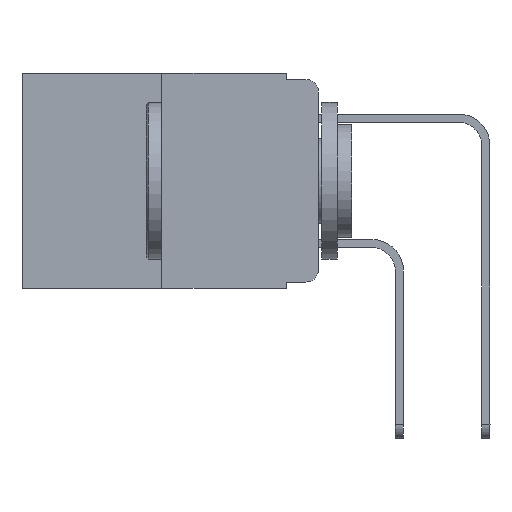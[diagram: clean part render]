
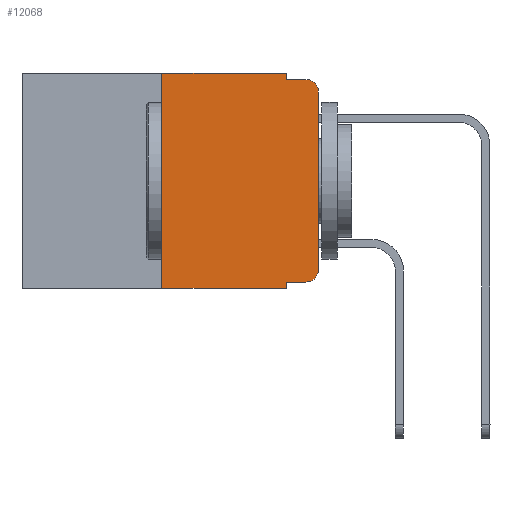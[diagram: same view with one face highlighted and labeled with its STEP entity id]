
A CAD part, left-side view. The second image highlights one B-rep face of the part: STEP entity #12068.
In plain terms, the highlighted planar face has unit normal (-1, 0, 0).
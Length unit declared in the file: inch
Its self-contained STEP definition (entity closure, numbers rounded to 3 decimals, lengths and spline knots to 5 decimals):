
#347 = CARTESIAN_POINT ( 'NONE',  ( 0., 0.051, -0.333 ) ) ;
#565 = LINE ( 'NONE', #16123, #12153 ) ;
#1091 = VERTEX_POINT ( 'NONE', #13543 ) ;
#1980 = DIRECTION ( 'NONE',  ( 0., 0., 1. ) ) ;
#3019 = DIRECTION ( 'NONE',  ( 0., 0., -1. ) ) ;
#3203 = PLANE ( 'NONE',  #16702 ) ;
#3685 = CARTESIAN_POINT ( 'NONE',  ( 0., 0.25, -0.343 ) ) ;
#3881 = DIRECTION ( 'NONE',  ( 0., 0., -1. ) ) ;
#3981 = ORIENTED_EDGE ( 'NONE', *, *, #6741, .F. ) ;
#4065 = VERTEX_POINT ( 'NONE', #16613 ) ;
#4074 = ORIENTED_EDGE ( 'NONE', *, *, #12992, .T. ) ;
#4576 = LINE ( 'NONE', #9655, #13757 ) ;
#4773 = ORIENTED_EDGE ( 'NONE', *, *, #21203, .T. ) ;
#4816 = AXIS2_PLACEMENT_3D ( 'NONE', #17775, #5701, #12593 ) ;
#5141 = CARTESIAN_POINT ( 'NONE',  ( 0., 0.02, -0.03 ) ) ;
#5701 = DIRECTION ( 'NONE',  ( -1., 0., 0. ) ) ;
#5902 = CARTESIAN_POINT ( 'NONE',  ( 0., 0.051, 0. ) ) ;
#6232 = VECTOR ( 'NONE', #3881, 39.37008 ) ;
#6681 = CARTESIAN_POINT ( 'NONE',  ( 0., 0., -0.313 ) ) ;
#6741 = EDGE_CURVE ( 'NONE', #17624, #17523, #10000, .T. ) ;
#6816 = ORIENTED_EDGE ( 'NONE', *, *, #11770, .F. ) ;
#6905 = DIRECTION ( 'NONE',  ( 0., 0., 1. ) ) ;
#7124 = CARTESIAN_POINT ( 'NONE',  ( 0., 0.25, 0. ) ) ;
#7152 = DIRECTION ( 'NONE',  ( 0., 0., -1. ) ) ;
#7201 = DIRECTION ( 'NONE',  ( 0., -1., 0. ) ) ;
#7350 = CIRCLE ( 'NONE', #18158, 0.02 ) ;
#7431 = DIRECTION ( 'NONE',  ( 0., -1., 0. ) ) ;
#8595 = DIRECTION ( 'NONE',  ( 0., 0., -1. ) ) ;
#8667 = ORIENTED_EDGE ( 'NONE', *, *, #10256, .F. ) ;
#8721 = ORIENTED_EDGE ( 'NONE', *, *, #20007, .T. ) ;
#8734 = EDGE_CURVE ( 'NONE', #21818, #17624, #14122, .T. ) ;
#8850 = DIRECTION ( 'NONE',  ( -1., 0., 0. ) ) ;
#9495 = ORIENTED_EDGE ( 'NONE', *, *, #8734, .F. ) ;
#9655 = CARTESIAN_POINT ( 'NONE',  ( 0., 0.051, -0.01 ) ) ;
#9665 = CARTESIAN_POINT ( 'NONE',  ( 0., 0., -0.03 ) ) ;
#9929 = VECTOR ( 'NONE', #1980, 39.37008 ) ;
#9994 = DIRECTION ( 'NONE',  ( 0., -1., 0. ) ) ;
#10000 = LINE ( 'NONE', #16873, #20249 ) ;
#10256 = EDGE_CURVE ( 'NONE', #12891, #20138, #4576, .T. ) ;
#10450 = VECTOR ( 'NONE', #6905, 39.37008 ) ;
#11178 = CARTESIAN_POINT ( 'NONE',  ( 0., 0.051, -0.333 ) ) ;
#11506 = VERTEX_POINT ( 'NONE', #9665 ) ;
#11571 = LINE ( 'NONE', #18458, #13852 ) ;
#11671 = DIRECTION ( 'NONE',  ( 0., -1., 0. ) ) ;
#11770 = EDGE_CURVE ( 'NONE', #12406, #1091, #12447, .T. ) ;
#12068 = ADVANCED_FACE ( 'NONE', ( #18648 ), #3203, .F. ) ;
#12153 = VECTOR ( 'NONE', #7431, 39.37008 ) ;
#12406 = VERTEX_POINT ( 'NONE', #11178 ) ;
#12447 = LINE ( 'NONE', #5902, #6232 ) ;
#12479 = VECTOR ( 'NONE', #7201, 39.37008 ) ;
#12593 = DIRECTION ( 'NONE',  ( 0., 0., -1. ) ) ;
#12862 = EDGE_CURVE ( 'NONE', #17523, #12891, #11571, .T. ) ;
#12891 = VERTEX_POINT ( 'NONE', #13718 ) ;
#12992 = EDGE_CURVE ( 'NONE', #11506, #20138, #7350, .T. ) ;
#13543 = CARTESIAN_POINT ( 'NONE',  ( 0., 0.051, -0.343 ) ) ;
#13711 = CARTESIAN_POINT ( 'NONE',  ( 0., 0., 0. ) ) ;
#13718 = CARTESIAN_POINT ( 'NONE',  ( 0., 0.051, -0.01 ) ) ;
#13757 = VECTOR ( 'NONE', #9994, 39.37008 ) ;
#13797 = CARTESIAN_POINT ( 'NONE',  ( 0., 0.473, 0. ) ) ;
#13852 = VECTOR ( 'NONE', #3019, 39.37008 ) ;
#13898 = DIRECTION ( 'NONE',  ( 1., 0., 0. ) ) ;
#14122 = LINE ( 'NONE', #7124, #10450 ) ;
#14223 = EDGE_LOOP ( 'NONE', ( #17016, #4074, #8667, #16635, #3981, #9495, #4773, #6816, #8721, #17682 ) ) ;
#15985 = EDGE_CURVE ( 'NONE', #4065, #19404, #20661, .T. ) ;
#16123 = CARTESIAN_POINT ( 'NONE',  ( 0., 0.473, -0.343 ) ) ;
#16548 = CARTESIAN_POINT ( 'NONE',  ( 0., 0.02, -0.01 ) ) ;
#16613 = CARTESIAN_POINT ( 'NONE',  ( 0., 0.02, -0.333 ) ) ;
#16635 = ORIENTED_EDGE ( 'NONE', *, *, #12862, .F. ) ;
#16702 = AXIS2_PLACEMENT_3D ( 'NONE', #13797, #13898, #8595 ) ;
#16873 = CARTESIAN_POINT ( 'NONE',  ( 0., 0.473, 0. ) ) ;
#17016 = ORIENTED_EDGE ( 'NONE', *, *, #19058, .T. ) ;
#17420 = LINE ( 'NONE', #13711, #9929 ) ;
#17523 = VERTEX_POINT ( 'NONE', #20143 ) ;
#17624 = VERTEX_POINT ( 'NONE', #18107 ) ;
#17682 = ORIENTED_EDGE ( 'NONE', *, *, #15985, .T. ) ;
#17775 = CARTESIAN_POINT ( 'NONE',  ( 0., 0.02, -0.313 ) ) ;
#18107 = CARTESIAN_POINT ( 'NONE',  ( 0., 0.25, 0. ) ) ;
#18158 = AXIS2_PLACEMENT_3D ( 'NONE', #5141, #8850, #7152 ) ;
#18458 = CARTESIAN_POINT ( 'NONE',  ( 0., 0.051, 0. ) ) ;
#18648 = FACE_OUTER_BOUND ( 'NONE', #14223, .T. ) ;
#19058 = EDGE_CURVE ( 'NONE', #19404, #11506, #17420, .T. ) ;
#19166 = LINE ( 'NONE', #347, #12479 ) ;
#19404 = VERTEX_POINT ( 'NONE', #6681 ) ;
#20007 = EDGE_CURVE ( 'NONE', #12406, #4065, #19166, .T. ) ;
#20138 = VERTEX_POINT ( 'NONE', #16548 ) ;
#20143 = CARTESIAN_POINT ( 'NONE',  ( 0., 0.051, 0. ) ) ;
#20249 = VECTOR ( 'NONE', #11671, 39.37008 ) ;
#20661 = CIRCLE ( 'NONE', #4816, 0.02 ) ;
#21203 = EDGE_CURVE ( 'NONE', #21818, #1091, #565, .T. ) ;
#21818 = VERTEX_POINT ( 'NONE', #3685 ) ;
